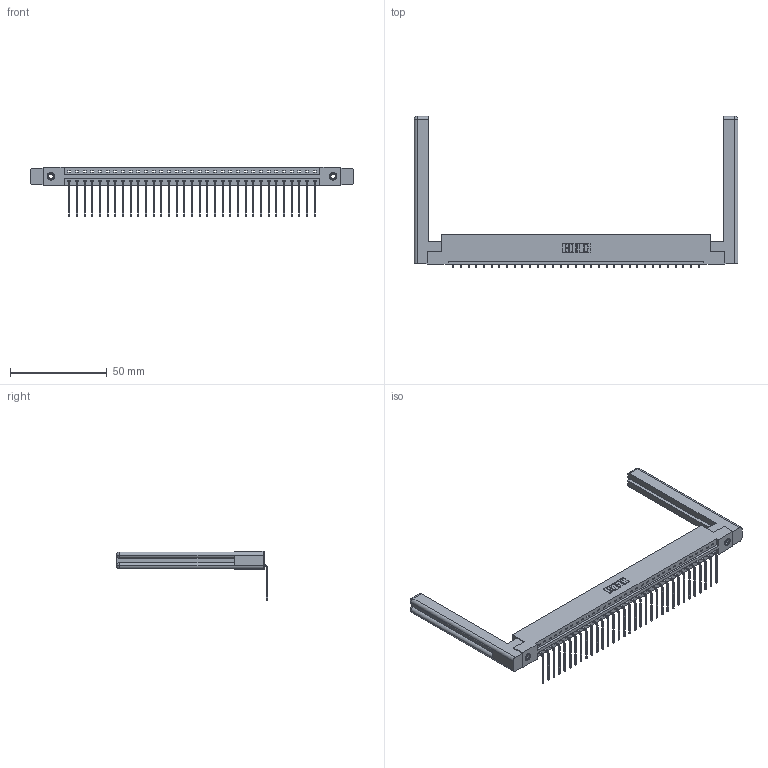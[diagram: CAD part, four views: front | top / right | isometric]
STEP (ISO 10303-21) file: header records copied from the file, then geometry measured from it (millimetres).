
FILE_DESCRIPTION (( 'STEP AP203' ), '1' );
FILE_NAME ('337-033-559-158.STEP', '2019-10-01T11:10:59', ( '' ), ( '' ), 'SwSTEP 2.0', 'SolidWorks 2016', '' );
FILE_SCHEMA (( 'CONFIG_CONTROL_DESIGN' ));
Length unit declared in the file: inch
Products named in the file (5): 307-220-058; 345-292-001_558 559 Tail - 1; 337 Part_Flush Mounting Lugs - 0.156 Dia-TI; 345-250-001_345-250-001-102; 337-033-559-158
Assembly tree (38 placements, depth 2):
  337-033-559-158
    337 Part_Flush Mounting Lugs - 0.156 Dia-TI
    345-292-001_558 559 Tail - 1  x33
    345-250-001_345-250-001-102  x2
    307-220-058  x2
Bounding box: 167.39 x 78.17 x 25.53 mm (x, y, z)
Volume: 24556.4 mm3; surface area: 23813 mm2
Topology: 38 solids, 38 shells, 2368 faces, 7067 edges, 4654 vertices
Faces by surface type: plane 1738, cylinder 606, cone 12, torus 12
Entity records: 28412 total; most frequent: CARTESIAN_POINT 4948, ORIENTED_EDGE 4856, DIRECTION 4202, EDGE_CURVE 2428, VECTOR 2252, LINE 2252, VERTEX_POINT 1610, AXIS2_PLACEMENT_3D 975
